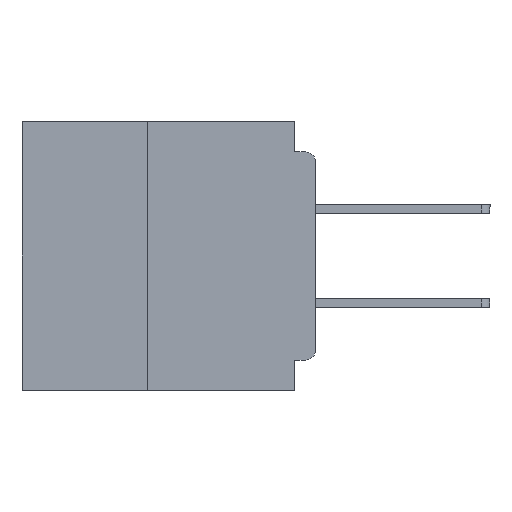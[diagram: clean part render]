
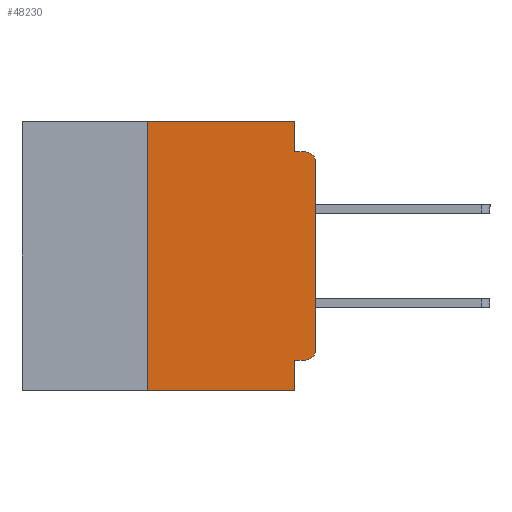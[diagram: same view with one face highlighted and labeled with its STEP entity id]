
A CAD part, left-side view. The second image highlights one B-rep face of the part: STEP entity #48230.
In plain terms, the highlighted planar face has unit normal (-1, 0, 0).
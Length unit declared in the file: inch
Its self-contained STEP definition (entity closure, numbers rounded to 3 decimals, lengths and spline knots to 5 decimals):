
#245 = DIRECTION ( 'NONE',  ( -1., 0., 0. ) ) ;
#426 = EDGE_CURVE ( 'NONE', #47809, #22274, #2538, .T. ) ;
#798 = CARTESIAN_POINT ( 'NONE',  ( 0., 0., -0.06 ) ) ;
#1203 = ORIENTED_EDGE ( 'NONE', *, *, #38057, .T. ) ;
#1269 = VECTOR ( 'NONE', #35799, 39.37008 ) ;
#1964 = VERTEX_POINT ( 'NONE', #39462 ) ;
#2061 = ORIENTED_EDGE ( 'NONE', *, *, #10685, .F. ) ;
#2538 = LINE ( 'NONE', #14576, #14378 ) ;
#4138 = EDGE_CURVE ( 'NONE', #12776, #47809, #56827, .T. ) ;
#4352 = EDGE_LOOP ( 'NONE', ( #21575, #1203, #22209, #20135, #57057, #44269, #42649, #2061, #38730, #24861 ) ) ;
#4692 = CARTESIAN_POINT ( 'NONE',  ( 0., 0.031, 0. ) ) ;
#5334 = CARTESIAN_POINT ( 'NONE',  ( 0., 0., -0.045 ) ) ;
#5844 = DIRECTION ( 'NONE',  ( 0., -1., 0. ) ) ;
#5870 = CARTESIAN_POINT ( 'NONE',  ( 0., 0.437, 0. ) ) ;
#8015 = LINE ( 'NONE', #5334, #19940 ) ;
#10685 = EDGE_CURVE ( 'NONE', #36118, #51847, #12548, .T. ) ;
#10906 = CARTESIAN_POINT ( 'NONE',  ( 0., 0.031, 0. ) ) ;
#11809 = EDGE_CURVE ( 'NONE', #49966, #15009, #35321, .T. ) ;
#12367 = CARTESIAN_POINT ( 'NONE',  ( 0., 0.437, 0. ) ) ;
#12476 = LINE ( 'NONE', #14947, #21562 ) ;
#12490 = DIRECTION ( 'NONE',  ( 0., 0., 1. ) ) ;
#12548 = LINE ( 'NONE', #40751, #34764 ) ;
#12600 = CARTESIAN_POINT ( 'NONE',  ( 0., 0.031, -0.045 ) ) ;
#12776 = VERTEX_POINT ( 'NONE', #49802 ) ;
#14373 = CARTESIAN_POINT ( 'NONE',  ( 0., 0.015, -0.34 ) ) ;
#14378 = VECTOR ( 'NONE', #16785, 39.37008 ) ;
#14576 = CARTESIAN_POINT ( 'NONE',  ( 0., 0., 0. ) ) ;
#14947 = CARTESIAN_POINT ( 'NONE',  ( 0., 0., -0.355 ) ) ;
#15009 = VERTEX_POINT ( 'NONE', #12600 ) ;
#16785 = DIRECTION ( 'NONE',  ( 0., 0., 1. ) ) ;
#16876 = DIRECTION ( 'NONE',  ( 0., -1., 0. ) ) ;
#17019 = CARTESIAN_POINT ( 'NONE',  ( 0., 0.25, -0.4 ) ) ;
#18879 = DIRECTION ( 'NONE',  ( 0., 0., -1. ) ) ;
#19359 = PLANE ( 'NONE',  #44824 ) ;
#19940 = VECTOR ( 'NONE', #36234, 39.37008 ) ;
#20135 = ORIENTED_EDGE ( 'NONE', *, *, #11809, .F. ) ;
#20751 = CIRCLE ( 'NONE', #31083, 0.015 ) ;
#21562 = VECTOR ( 'NONE', #41474, 39.37008 ) ;
#21575 = ORIENTED_EDGE ( 'NONE', *, *, #426, .T. ) ;
#22209 = ORIENTED_EDGE ( 'NONE', *, *, #39144, .F. ) ;
#22274 = VERTEX_POINT ( 'NONE', #798 ) ;
#22513 = LINE ( 'NONE', #17019, #32872 ) ;
#23806 = DIRECTION ( 'NONE',  ( 0., 0., -1. ) ) ;
#24059 = FACE_OUTER_BOUND ( 'NONE', #4352, .T. ) ;
#24431 = LINE ( 'NONE', #32469, #37567 ) ;
#24861 = ORIENTED_EDGE ( 'NONE', *, *, #4138, .T. ) ;
#25021 = CARTESIAN_POINT ( 'NONE',  ( 0., 0., -0.34 ) ) ;
#26189 = EDGE_CURVE ( 'NONE', #12776, #36118, #12476, .T. ) ;
#26925 = CARTESIAN_POINT ( 'NONE',  ( 0., 0.015, -0.06 ) ) ;
#27743 = EDGE_CURVE ( 'NONE', #51375, #49966, #41425, .T. ) ;
#29672 = EDGE_CURVE ( 'NONE', #47197, #51375, #22513, .T. ) ;
#31083 = AXIS2_PLACEMENT_3D ( 'NONE', #26925, #245, #31338 ) ;
#31338 = DIRECTION ( 'NONE',  ( 0., 0., -1. ) ) ;
#32469 = CARTESIAN_POINT ( 'NONE',  ( 0., 0.437, -0.4 ) ) ;
#32872 = VECTOR ( 'NONE', #12490, 39.37008 ) ;
#34020 = CARTESIAN_POINT ( 'NONE',  ( 0., 0.25, 0. ) ) ;
#34764 = VECTOR ( 'NONE', #53814, 39.37008 ) ;
#35321 = LINE ( 'NONE', #4692, #1269 ) ;
#35799 = DIRECTION ( 'NONE',  ( 0., 0., -1. ) ) ;
#36118 = VERTEX_POINT ( 'NONE', #39482 ) ;
#36234 = DIRECTION ( 'NONE',  ( 0., -1., 0. ) ) ;
#37567 = VECTOR ( 'NONE', #5844, 39.37008 ) ;
#38057 = EDGE_CURVE ( 'NONE', #22274, #1964, #20751, .T. ) ;
#38730 = ORIENTED_EDGE ( 'NONE', *, *, #26189, .F. ) ;
#39144 = EDGE_CURVE ( 'NONE', #15009, #1964, #8015, .T. ) ;
#39462 = CARTESIAN_POINT ( 'NONE',  ( 0., 0.015, -0.045 ) ) ;
#39482 = CARTESIAN_POINT ( 'NONE',  ( 0., 0.031, -0.355 ) ) ;
#40751 = CARTESIAN_POINT ( 'NONE',  ( 0., 0.031, -0.4 ) ) ;
#41425 = LINE ( 'NONE', #12367, #51753 ) ;
#41474 = DIRECTION ( 'NONE',  ( 0., 1., 0. ) ) ;
#41530 = CARTESIAN_POINT ( 'NONE',  ( 0., 0.031, -0.4 ) ) ;
#42649 = ORIENTED_EDGE ( 'NONE', *, *, #44466, .T. ) ;
#44269 = ORIENTED_EDGE ( 'NONE', *, *, #29672, .F. ) ;
#44466 = EDGE_CURVE ( 'NONE', #47197, #51847, #24431, .T. ) ;
#44824 = AXIS2_PLACEMENT_3D ( 'NONE', #5870, #50256, #23806 ) ;
#45356 = DIRECTION ( 'NONE',  ( -1., 0., 0. ) ) ;
#47197 = VERTEX_POINT ( 'NONE', #50961 ) ;
#47809 = VERTEX_POINT ( 'NONE', #25021 ) ;
#48230 = ADVANCED_FACE ( 'NONE', ( #24059 ), #19359, .F. ) ;
#49617 = AXIS2_PLACEMENT_3D ( 'NONE', #14373, #45356, #18879 ) ;
#49802 = CARTESIAN_POINT ( 'NONE',  ( 0., 0.015, -0.355 ) ) ;
#49966 = VERTEX_POINT ( 'NONE', #10906 ) ;
#50256 = DIRECTION ( 'NONE',  ( 1., 0., 0. ) ) ;
#50961 = CARTESIAN_POINT ( 'NONE',  ( 0., 0.25, -0.4 ) ) ;
#51375 = VERTEX_POINT ( 'NONE', #34020 ) ;
#51753 = VECTOR ( 'NONE', #16876, 39.37008 ) ;
#51847 = VERTEX_POINT ( 'NONE', #41530 ) ;
#53814 = DIRECTION ( 'NONE',  ( 0., 0., -1. ) ) ;
#56827 = CIRCLE ( 'NONE', #49617, 0.015 ) ;
#57057 = ORIENTED_EDGE ( 'NONE', *, *, #27743, .F. ) ;
